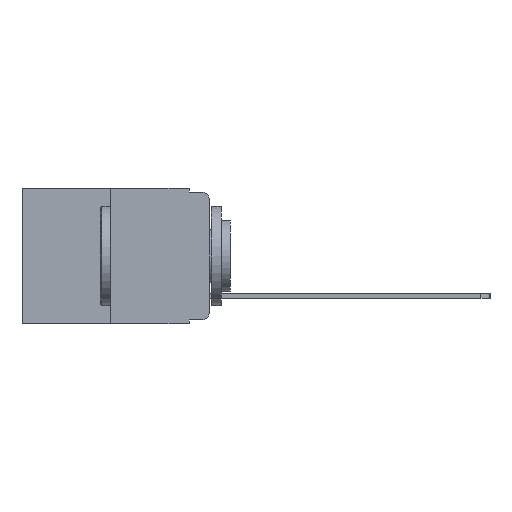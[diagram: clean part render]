
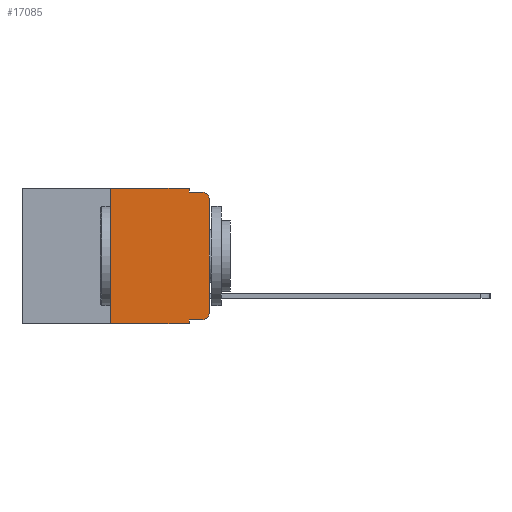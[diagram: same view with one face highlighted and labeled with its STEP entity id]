
A CAD part, left-side view. The second image highlights one B-rep face of the part: STEP entity #17085.
In plain terms, the highlighted planar face has unit normal (-1, 0, 0).
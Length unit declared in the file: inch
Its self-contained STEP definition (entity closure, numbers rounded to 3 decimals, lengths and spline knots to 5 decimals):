
#116 = CARTESIAN_POINT ( 'NONE',  ( 0., 0.051, -0.333 ) ) ;
#209 = DIRECTION ( 'NONE',  ( -1., 0., 0. ) ) ;
#313 = DIRECTION ( 'NONE',  ( 0., 0., -1. ) ) ;
#433 = EDGE_CURVE ( 'NONE', #17457, #13237, #7076, .T. ) ;
#484 = CARTESIAN_POINT ( 'NONE',  ( 0., 0.051, -0.01 ) ) ;
#701 = DIRECTION ( 'NONE',  ( 0., -1., 0. ) ) ;
#927 = AXIS2_PLACEMENT_3D ( 'NONE', #2532, #2113, #3755 ) ;
#1269 = LINE ( 'NONE', #20170, #11572 ) ;
#1351 = CARTESIAN_POINT ( 'NONE',  ( 0., 0.473, 0. ) ) ;
#1623 = CARTESIAN_POINT ( 'NONE',  ( 0., 0.25, 0. ) ) ;
#1639 = ORIENTED_EDGE ( 'NONE', *, *, #12769, .F. ) ;
#1804 = EDGE_CURVE ( 'NONE', #6345, #17457, #9353, .T. ) ;
#1850 = EDGE_CURVE ( 'NONE', #12488, #5730, #14621, .T. ) ;
#1915 = PLANE ( 'NONE',  #13260 ) ;
#2025 = LINE ( 'NONE', #25035, #12303 ) ;
#2113 = DIRECTION ( 'NONE',  ( -1., 0., 0. ) ) ;
#2530 = EDGE_CURVE ( 'NONE', #20896, #12475, #23775, .T. ) ;
#2532 = CARTESIAN_POINT ( 'NONE',  ( 0., 0.02, -0.313 ) ) ;
#3278 = ORIENTED_EDGE ( 'NONE', *, *, #3943, .T. ) ;
#3513 = LINE ( 'NONE', #22843, #24016 ) ;
#3755 = DIRECTION ( 'NONE',  ( 0., 0., -1. ) ) ;
#3893 = VECTOR ( 'NONE', #701, 39.37008 ) ;
#3943 = EDGE_CURVE ( 'NONE', #13237, #20896, #23699, .T. ) ;
#4025 = CARTESIAN_POINT ( 'NONE',  ( 0., 0.473, 0. ) ) ;
#4557 = ORIENTED_EDGE ( 'NONE', *, *, #9953, .F. ) ;
#5288 = DIRECTION ( 'NONE',  ( 0., 0., 1. ) ) ;
#5661 = AXIS2_PLACEMENT_3D ( 'NONE', #12469, #209, #313 ) ;
#5730 = VERTEX_POINT ( 'NONE', #9416 ) ;
#6112 = DIRECTION ( 'NONE',  ( 1., 0., 0. ) ) ;
#6345 = VERTEX_POINT ( 'NONE', #116 ) ;
#7076 = CIRCLE ( 'NONE', #927, 0.02 ) ;
#7126 = CARTESIAN_POINT ( 'NONE',  ( 0., 0.051, 0. ) ) ;
#8377 = CARTESIAN_POINT ( 'NONE',  ( 0., 0., -0.03 ) ) ;
#8732 = ORIENTED_EDGE ( 'NONE', *, *, #2530, .T. ) ;
#8775 = CARTESIAN_POINT ( 'NONE',  ( 0., 0., -0.313 ) ) ;
#9170 = DIRECTION ( 'NONE',  ( 0., 0., -1. ) ) ;
#9172 = CARTESIAN_POINT ( 'NONE',  ( 0., 0.051, -0.333 ) ) ;
#9353 = LINE ( 'NONE', #9172, #3893 ) ;
#9415 = VERTEX_POINT ( 'NONE', #24263 ) ;
#9416 = CARTESIAN_POINT ( 'NONE',  ( 0., 0.051, -0.343 ) ) ;
#9953 = EDGE_CURVE ( 'NONE', #9415, #24230, #1269, .T. ) ;
#10024 = ORIENTED_EDGE ( 'NONE', *, *, #18732, .F. ) ;
#10402 = DIRECTION ( 'NONE',  ( 0., 0., -1. ) ) ;
#11304 = ORIENTED_EDGE ( 'NONE', *, *, #14058, .F. ) ;
#11572 = VECTOR ( 'NONE', #10402, 39.37008 ) ;
#12187 = CARTESIAN_POINT ( 'NONE',  ( 0., 0.25, -0.343 ) ) ;
#12303 = VECTOR ( 'NONE', #15335, 39.37008 ) ;
#12469 = CARTESIAN_POINT ( 'NONE',  ( 0., 0.02, -0.03 ) ) ;
#12475 = VERTEX_POINT ( 'NONE', #16014 ) ;
#12488 = VERTEX_POINT ( 'NONE', #12187 ) ;
#12769 = EDGE_CURVE ( 'NONE', #6345, #5730, #14781, .T. ) ;
#13022 = DIRECTION ( 'NONE',  ( 0., -1., 0. ) ) ;
#13237 = VERTEX_POINT ( 'NONE', #8775 ) ;
#13260 = AXIS2_PLACEMENT_3D ( 'NONE', #4025, #6112, #19998 ) ;
#13402 = VECTOR ( 'NONE', #13022, 39.37008 ) ;
#14058 = EDGE_CURVE ( 'NONE', #12488, #25591, #2025, .T. ) ;
#14621 = LINE ( 'NONE', #21123, #13402 ) ;
#14781 = LINE ( 'NONE', #7126, #24523 ) ;
#15335 = DIRECTION ( 'NONE',  ( 0., 0., 1. ) ) ;
#15529 = DIRECTION ( 'NONE',  ( 0., -1., 0. ) ) ;
#16014 = CARTESIAN_POINT ( 'NONE',  ( 0., 0.02, -0.01 ) ) ;
#16489 = ORIENTED_EDGE ( 'NONE', *, *, #1850, .T. ) ;
#17059 = DIRECTION ( 'NONE',  ( 0., -1., 0. ) ) ;
#17085 = ADVANCED_FACE ( 'NONE', ( #21872 ), #1915, .F. ) ;
#17457 = VERTEX_POINT ( 'NONE', #24970 ) ;
#18348 = ORIENTED_EDGE ( 'NONE', *, *, #1804, .T. ) ;
#18732 = EDGE_CURVE ( 'NONE', #25591, #9415, #25165, .T. ) ;
#19233 = CARTESIAN_POINT ( 'NONE',  ( 0., 0., 0. ) ) ;
#19567 = ORIENTED_EDGE ( 'NONE', *, *, #433, .T. ) ;
#19853 = ORIENTED_EDGE ( 'NONE', *, *, #20485, .F. ) ;
#19998 = DIRECTION ( 'NONE',  ( 0., 0., -1. ) ) ;
#20020 = VECTOR ( 'NONE', #15529, 39.37008 ) ;
#20170 = CARTESIAN_POINT ( 'NONE',  ( 0., 0.051, 0. ) ) ;
#20485 = EDGE_CURVE ( 'NONE', #24230, #12475, #3513, .T. ) ;
#20896 = VERTEX_POINT ( 'NONE', #8377 ) ;
#21123 = CARTESIAN_POINT ( 'NONE',  ( 0., 0.473, -0.343 ) ) ;
#21872 = FACE_OUTER_BOUND ( 'NONE', #22893, .T. ) ;
#22843 = CARTESIAN_POINT ( 'NONE',  ( 0., 0.051, -0.01 ) ) ;
#22893 = EDGE_LOOP ( 'NONE', ( #3278, #8732, #19853, #4557, #10024, #11304, #16489, #1639, #18348, #19567 ) ) ;
#23101 = VECTOR ( 'NONE', #5288, 39.37008 ) ;
#23699 = LINE ( 'NONE', #19233, #23101 ) ;
#23775 = CIRCLE ( 'NONE', #5661, 0.02 ) ;
#24016 = VECTOR ( 'NONE', #17059, 39.37008 ) ;
#24230 = VERTEX_POINT ( 'NONE', #484 ) ;
#24263 = CARTESIAN_POINT ( 'NONE',  ( 0., 0.051, 0. ) ) ;
#24523 = VECTOR ( 'NONE', #9170, 39.37008 ) ;
#24970 = CARTESIAN_POINT ( 'NONE',  ( 0., 0.02, -0.333 ) ) ;
#25035 = CARTESIAN_POINT ( 'NONE',  ( 0., 0.25, 0. ) ) ;
#25165 = LINE ( 'NONE', #1351, #20020 ) ;
#25591 = VERTEX_POINT ( 'NONE', #1623 ) ;
